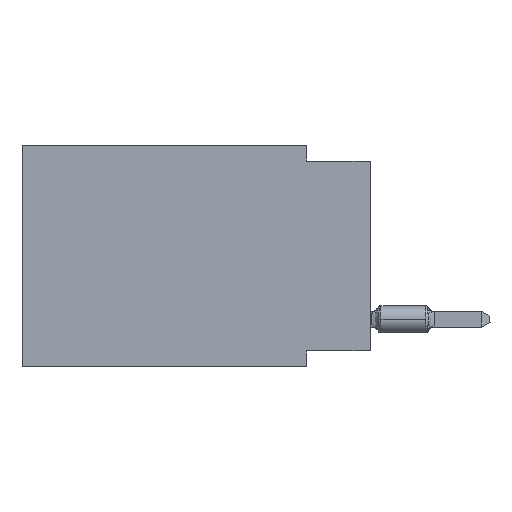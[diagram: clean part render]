
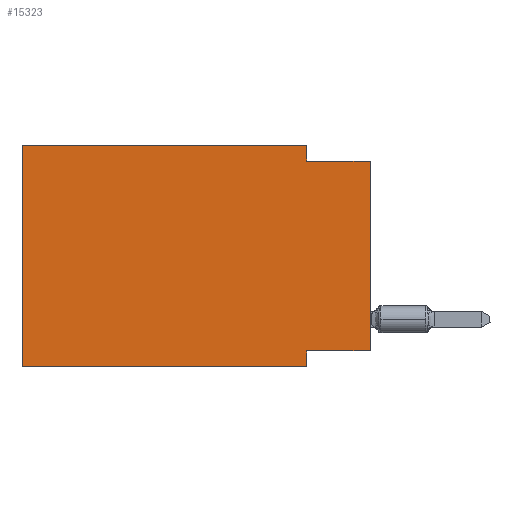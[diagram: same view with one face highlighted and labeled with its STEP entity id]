
A CAD part, left-side view. The second image highlights one B-rep face of the part: STEP entity #15323.
In plain terms, the highlighted planar face has unit normal (-1, 0, 0).
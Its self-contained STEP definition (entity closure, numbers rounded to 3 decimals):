
#1656 = CARTESIAN_POINT ( 'NONE',  ( 0., 13.97, 0. ) ) ;
#2302 = ORIENTED_EDGE ( 'NONE', *, *, #65644, .T. ) ;
#2746 = EDGE_CURVE ( 'NONE', #3914, #5382, #34701, .T. ) ;
#2874 = DIRECTION ( 'NONE',  ( 0., 1., 0. ) ) ;
#3206 = VECTOR ( 'NONE', #39374, 1000. ) ;
#3209 = ORIENTED_EDGE ( 'NONE', *, *, #27531, .F. ) ;
#3914 = VERTEX_POINT ( 'NONE', #51425 ) ;
#5212 = ORIENTED_EDGE ( 'NONE', *, *, #33657, .F. ) ;
#5382 = VERTEX_POINT ( 'NONE', #10088 ) ;
#6516 = DIRECTION ( 'NONE',  ( 0., -1., 0. ) ) ;
#7217 = LINE ( 'NONE', #50807, #8672 ) ;
#8672 = VECTOR ( 'NONE', #6516, 1000. ) ;
#10088 = CARTESIAN_POINT ( 'NONE',  ( 0., 2.54, -8.255 ) ) ;
#10264 = VECTOR ( 'NONE', #64706, 1000. ) ;
#10491 = VERTEX_POINT ( 'NONE', #21022 ) ;
#11251 = CARTESIAN_POINT ( 'NONE',  ( 0., 0., -0.635 ) ) ;
#12307 = CARTESIAN_POINT ( 'NONE',  ( 0., 13.97, -8.89 ) ) ;
#13616 = CARTESIAN_POINT ( 'NONE',  ( 0., 0., -8.255 ) ) ;
#13863 = CARTESIAN_POINT ( 'NONE',  ( 0., 13.97, 0. ) ) ;
#14476 = EDGE_CURVE ( 'NONE', #28758, #27169, #62803, .T. ) ;
#15323 = ADVANCED_FACE ( 'NONE', ( #18901 ), #47102, .F. ) ;
#18901 = FACE_OUTER_BOUND ( 'NONE', #30850, .T. ) ;
#19564 = VERTEX_POINT ( 'NONE', #51767 ) ;
#19600 = DIRECTION ( 'NONE',  ( 1., 0., 0. ) ) ;
#19629 = CARTESIAN_POINT ( 'NONE',  ( 0., 2.54, -0.635 ) ) ;
#21022 = CARTESIAN_POINT ( 'NONE',  ( 0., 0., -0.635 ) ) ;
#21443 = ORIENTED_EDGE ( 'NONE', *, *, #68615, .F. ) ;
#21480 = CARTESIAN_POINT ( 'NONE',  ( 0., 0., 0. ) ) ;
#22319 = LINE ( 'NONE', #11251, #44303 ) ;
#22729 = VECTOR ( 'NONE', #60969, 1000. ) ;
#23653 = EDGE_CURVE ( 'NONE', #28758, #59857, #7217, .T. ) ;
#24596 = VECTOR ( 'NONE', #2874, 1000. ) ;
#27169 = VERTEX_POINT ( 'NONE', #1656 ) ;
#27531 = EDGE_CURVE ( 'NONE', #27169, #19564, #39847, .T. ) ;
#28758 = VERTEX_POINT ( 'NONE', #12307 ) ;
#29053 = ORIENTED_EDGE ( 'NONE', *, *, #2746, .F. ) ;
#30850 = EDGE_LOOP ( 'NONE', ( #2302, #21443, #67092, #3209, #43709, #69206, #5212, #29053 ) ) ;
#31534 = DIRECTION ( 'NONE',  ( 0., -1., 0. ) ) ;
#32953 = AXIS2_PLACEMENT_3D ( 'NONE', #40726, #19600, #56793 ) ;
#33657 = EDGE_CURVE ( 'NONE', #5382, #59857, #61498, .T. ) ;
#34701 = LINE ( 'NONE', #13616, #24596 ) ;
#35660 = DIRECTION ( 'NONE',  ( 0., 0., 1. ) ) ;
#35680 = VECTOR ( 'NONE', #31534, 1000. ) ;
#39374 = DIRECTION ( 'NONE',  ( 0., 0., -1. ) ) ;
#39847 = LINE ( 'NONE', #41943, #35680 ) ;
#40726 = CARTESIAN_POINT ( 'NONE',  ( 0., 13.97, 0. ) ) ;
#41943 = CARTESIAN_POINT ( 'NONE',  ( 0., 13.97, 0. ) ) ;
#43709 = ORIENTED_EDGE ( 'NONE', *, *, #14476, .F. ) ;
#44137 = DIRECTION ( 'NONE',  ( 0., -1., 0. ) ) ;
#44303 = VECTOR ( 'NONE', #44137, 1000. ) ;
#44895 = CARTESIAN_POINT ( 'NONE',  ( 0., 2.54, 0. ) ) ;
#44911 = EDGE_CURVE ( 'NONE', #19564, #47761, #51319, .T. ) ;
#47102 = PLANE ( 'NONE',  #32953 ) ;
#47761 = VERTEX_POINT ( 'NONE', #19629 ) ;
#50807 = CARTESIAN_POINT ( 'NONE',  ( 0., 13.97, -8.89 ) ) ;
#51319 = LINE ( 'NONE', #44895, #22729 ) ;
#51425 = CARTESIAN_POINT ( 'NONE',  ( 0., 0., -8.255 ) ) ;
#51542 = CARTESIAN_POINT ( 'NONE',  ( 0., 2.54, -8.89 ) ) ;
#51767 = CARTESIAN_POINT ( 'NONE',  ( 0., 2.54, 0. ) ) ;
#56793 = DIRECTION ( 'NONE',  ( 0., 0., -1. ) ) ;
#58972 = VECTOR ( 'NONE', #35660, 1000. ) ;
#59857 = VERTEX_POINT ( 'NONE', #51542 ) ;
#60969 = DIRECTION ( 'NONE',  ( 0., 0., -1. ) ) ;
#61498 = LINE ( 'NONE', #62201, #3206 ) ;
#62201 = CARTESIAN_POINT ( 'NONE',  ( 0., 2.54, -8.89 ) ) ;
#62803 = LINE ( 'NONE', #13863, #58972 ) ;
#64706 = DIRECTION ( 'NONE',  ( 0., 0., 1. ) ) ;
#65644 = EDGE_CURVE ( 'NONE', #3914, #10491, #69702, .T. ) ;
#67092 = ORIENTED_EDGE ( 'NONE', *, *, #44911, .F. ) ;
#68615 = EDGE_CURVE ( 'NONE', #47761, #10491, #22319, .T. ) ;
#69206 = ORIENTED_EDGE ( 'NONE', *, *, #23653, .T. ) ;
#69702 = LINE ( 'NONE', #21480, #10264 ) ;
